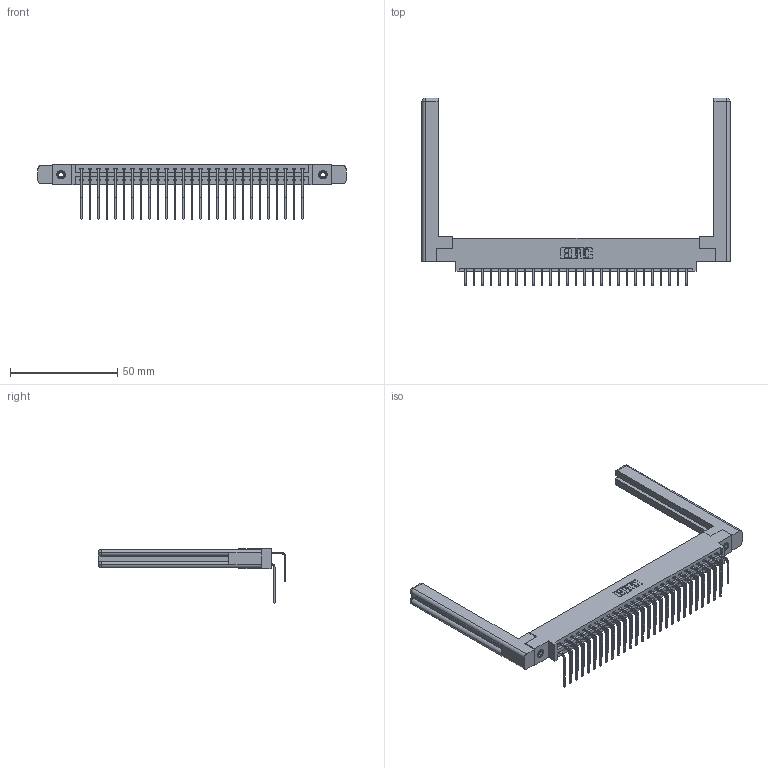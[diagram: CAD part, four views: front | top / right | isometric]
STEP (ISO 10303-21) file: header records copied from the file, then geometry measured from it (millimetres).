
FILE_DESCRIPTION (( 'STEP AP203' ), '1' );
FILE_NAME ('337-054-558-858.STEP', '2019-10-11T19:20:50', ( '' ), ( '' ), 'SwSTEP 2.0', 'SolidWorks 2016', '' );
FILE_SCHEMA (( 'CONFIG_CONTROL_DESIGN' ));
Length unit declared in the file: inch
Products named in the file (6): 345-250-001_345-250-001-102; 345-292-001_558 559 Tail - 1; 337-054-558-858; 337 Part_0.170 Offset - 0.156 Dia-TI; 345-292-001_558 Tail - 2; 307-220-058
Assembly tree (59 placements, depth 2):
  337-054-558-858
    337 Part_0.170 Offset - 0.156 Dia-TI
    345-292-001_558 559 Tail - 1  x27
    345-292-001_558 Tail - 2  x27
    345-250-001_345-250-001-102  x2
    307-220-058  x2
Bounding box: 143.61 x 87.57 x 25.53 mm (x, y, z)
Volume: 22271.6 mm3; surface area: 23676.7 mm2
Topology: 59 solids, 59 shells, 3284 faces, 9695 edges, 6378 vertices
Faces by surface type: plane 2318, cylinder 942, cone 12, torus 12
Entity records: 27424 total; most frequent: CARTESIAN_POINT 4688, ORIENTED_EDGE 4512, DIRECTION 4012, EDGE_CURVE 2256, VECTOR 2040, LINE 2040, VERTEX_POINT 1494, AXIS2_PLACEMENT_3D 986
